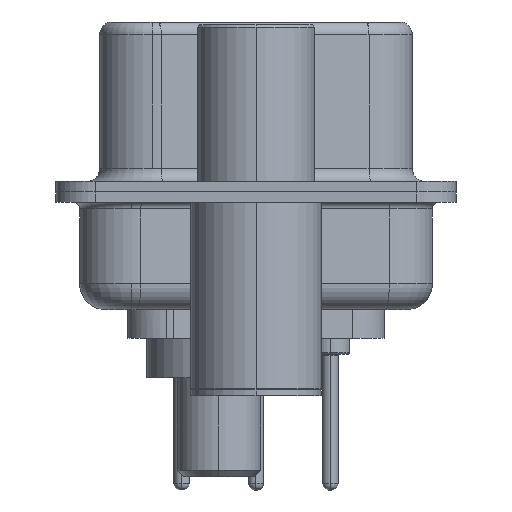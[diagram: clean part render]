
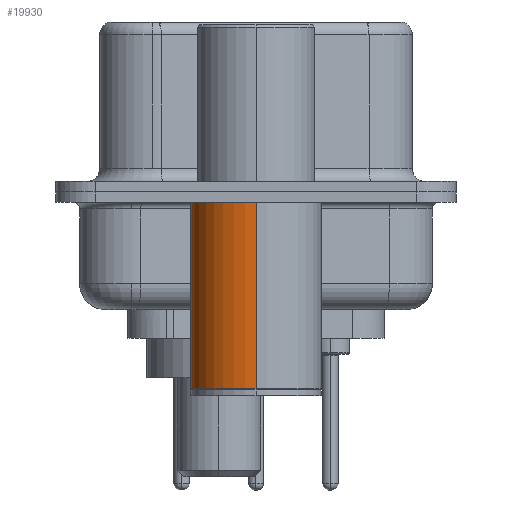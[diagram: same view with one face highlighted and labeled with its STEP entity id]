
A CAD part, left-side view. The second image highlights one B-rep face of the part: STEP entity #19930.
In plain terms, the highlighted cylindrical face has radius 2.5 mm (diameter 5 mm), a partial arc.
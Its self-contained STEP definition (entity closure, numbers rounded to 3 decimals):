
#1328 = CARTESIAN_POINT ( 'NONE',  ( -2.5, 0., -0.4 ) ) ;
#1555 = DIRECTION ( 'NONE',  ( 1., 0., 0. ) ) ;
#1653 = AXIS2_PLACEMENT_3D ( 'NONE', #10064, #28057, #12629 ) ;
#2050 = EDGE_CURVE ( 'NONE', #24255, #19882, #28397, .T. ) ;
#2124 = ORIENTED_EDGE ( 'NONE', *, *, #16885, .F. ) ;
#5572 = VECTOR ( 'NONE', #19294, 1000. ) ;
#6585 = AXIS2_PLACEMENT_3D ( 'NONE', #8943, #7617, #7507 ) ;
#7507 = DIRECTION ( 'NONE',  ( 1., 0., 0. ) ) ;
#7617 = DIRECTION ( 'NONE',  ( 0., 0., 1. ) ) ;
#8198 = CARTESIAN_POINT ( 'NONE',  ( -2.5, 0., 0.581 ) ) ;
#8943 = CARTESIAN_POINT ( 'NONE',  ( 0., 0., -7.525 ) ) ;
#9051 = CARTESIAN_POINT ( 'NONE',  ( 2.5, 0., 0.581 ) ) ;
#9878 = FACE_OUTER_BOUND ( 'NONE', #31658, .T. ) ;
#10064 = CARTESIAN_POINT ( 'NONE',  ( 0., 0., -0.4 ) ) ;
#11743 = CARTESIAN_POINT ( 'NONE',  ( 0., 0., 0.581 ) ) ;
#12629 = DIRECTION ( 'NONE',  ( 1., 0., 0. ) ) ;
#13254 = VECTOR ( 'NONE', #15445, 1000. ) ;
#13615 = ORIENTED_EDGE ( 'NONE', *, *, #2050, .T. ) ;
#14149 = VERTEX_POINT ( 'NONE', #1328 ) ;
#14194 = CARTESIAN_POINT ( 'NONE',  ( -2.5, 0., -7.525 ) ) ;
#14251 = CYLINDRICAL_SURFACE ( 'NONE', #14402, 2.5 ) ;
#14402 = AXIS2_PLACEMENT_3D ( 'NONE', #11743, #17056, #1555 ) ;
#15445 = DIRECTION ( 'NONE',  ( 0., 0., 1. ) ) ;
#16885 = EDGE_CURVE ( 'NONE', #24255, #17915, #19287, .T. ) ;
#17056 = DIRECTION ( 'NONE',  ( 0., 0., 1. ) ) ;
#17419 = ORIENTED_EDGE ( 'NONE', *, *, #26742, .T. ) ;
#17915 = VERTEX_POINT ( 'NONE', #28558 ) ;
#19287 = LINE ( 'NONE', #9051, #5572 ) ;
#19294 = DIRECTION ( 'NONE',  ( 0., 0., 1. ) ) ;
#19433 = CARTESIAN_POINT ( 'NONE',  ( 2.5, 0., -7.525 ) ) ;
#19882 = VERTEX_POINT ( 'NONE', #14194 ) ;
#19930 = ADVANCED_FACE ( 'NONE', ( #9878 ), #14251, .T. ) ;
#20108 = EDGE_CURVE ( 'NONE', #17915, #14149, #23938, .T. ) ;
#20138 = LINE ( 'NONE', #8198, #13254 ) ;
#23938 = CIRCLE ( 'NONE', #1653, 2.5 ) ;
#24255 = VERTEX_POINT ( 'NONE', #19433 ) ;
#26742 = EDGE_CURVE ( 'NONE', #19882, #14149, #20138, .T. ) ;
#28057 = DIRECTION ( 'NONE',  ( 0., 0., 1. ) ) ;
#28397 = CIRCLE ( 'NONE', #6585, 2.5 ) ;
#28558 = CARTESIAN_POINT ( 'NONE',  ( 2.5, 0., -0.4 ) ) ;
#30308 = ORIENTED_EDGE ( 'NONE', *, *, #20108, .F. ) ;
#31658 = EDGE_LOOP ( 'NONE', ( #13615, #17419, #30308, #2124 ) ) ;
